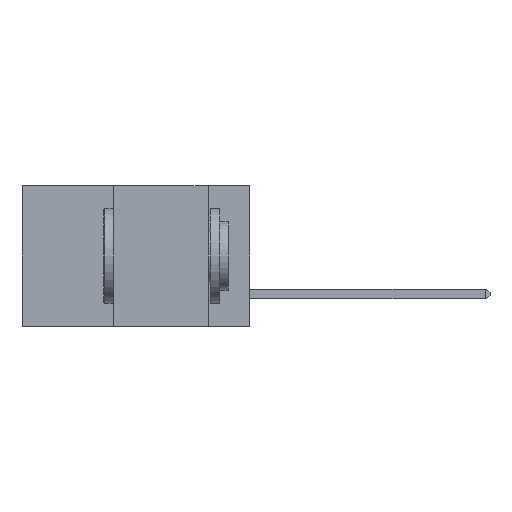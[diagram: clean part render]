
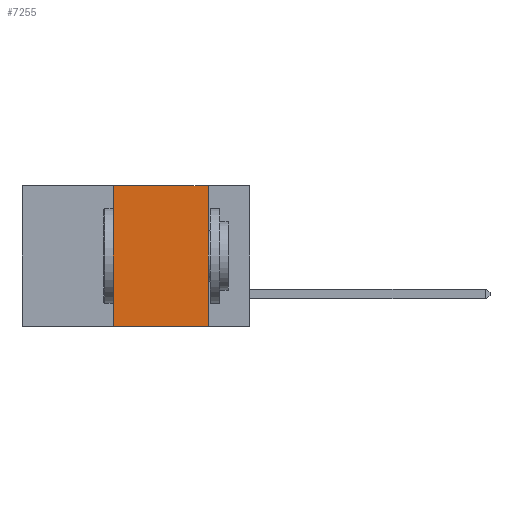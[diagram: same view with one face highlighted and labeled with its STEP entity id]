
A CAD part, left-side view. The second image highlights one B-rep face of the part: STEP entity #7255.
In plain terms, the highlighted planar face has unit normal (-1, 0, 0).
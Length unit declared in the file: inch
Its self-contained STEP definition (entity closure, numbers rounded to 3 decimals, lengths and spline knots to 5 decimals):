
#414 = CARTESIAN_POINT ( 'NONE',  ( 0., 0.11, 0. ) ) ;
#496 = VECTOR ( 'NONE', #1938, 39.37008 ) ;
#1371 = CARTESIAN_POINT ( 'NONE',  ( 0., 0.11, -0.37 ) ) ;
#1938 = DIRECTION ( 'NONE',  ( 0., -1., 0. ) ) ;
#4085 = EDGE_LOOP ( 'NONE', ( #32384, #26216, #20882, #34862 ) ) ;
#5533 = AXIS2_PLACEMENT_3D ( 'NONE', #5590, #24552, #8397 ) ;
#5590 = CARTESIAN_POINT ( 'NONE',  ( 0., 0.6, 0. ) ) ;
#5744 = VECTOR ( 'NONE', #29023, 39.37008 ) ;
#6778 = EDGE_CURVE ( 'NONE', #27101, #29954, #11664, .T. ) ;
#7187 = CARTESIAN_POINT ( 'NONE',  ( 0., 0.36, 0. ) ) ;
#7255 = ADVANCED_FACE ( 'NONE', ( #34595 ), #21906, .F. ) ;
#8397 = DIRECTION ( 'NONE',  ( 0., 0., -1. ) ) ;
#10654 = CARTESIAN_POINT ( 'NONE',  ( 0., 0.36, -0.37 ) ) ;
#11625 = VECTOR ( 'NONE', #34491, 39.37008 ) ;
#11664 = LINE ( 'NONE', #414, #18838 ) ;
#11683 = CARTESIAN_POINT ( 'NONE',  ( 0., 0.11, 0. ) ) ;
#11905 = EDGE_CURVE ( 'NONE', #31286, #27101, #13135, .T. ) ;
#13135 = LINE ( 'NONE', #20959, #5744 ) ;
#15729 = CARTESIAN_POINT ( 'NONE',  ( 0., 0.6, -0.37 ) ) ;
#18838 = VECTOR ( 'NONE', #30053, 39.37008 ) ;
#20882 = ORIENTED_EDGE ( 'NONE', *, *, #34337, .F. ) ;
#20959 = CARTESIAN_POINT ( 'NONE',  ( 0., 0.6, 0. ) ) ;
#21906 = PLANE ( 'NONE',  #5533 ) ;
#24552 = DIRECTION ( 'NONE',  ( 1., 0., 0. ) ) ;
#25136 = VERTEX_POINT ( 'NONE', #10654 ) ;
#26216 = ORIENTED_EDGE ( 'NONE', *, *, #11905, .F. ) ;
#27101 = VERTEX_POINT ( 'NONE', #11683 ) ;
#29023 = DIRECTION ( 'NONE',  ( 0., -1., 0. ) ) ;
#29954 = VERTEX_POINT ( 'NONE', #1371 ) ;
#30053 = DIRECTION ( 'NONE',  ( 0., 0., -1. ) ) ;
#31286 = VERTEX_POINT ( 'NONE', #7187 ) ;
#31848 = CARTESIAN_POINT ( 'NONE',  ( 0., 0.36, 0. ) ) ;
#32384 = ORIENTED_EDGE ( 'NONE', *, *, #6778, .F. ) ;
#32575 = EDGE_CURVE ( 'NONE', #25136, #29954, #34596, .T. ) ;
#32810 = LINE ( 'NONE', #31848, #11625 ) ;
#34337 = EDGE_CURVE ( 'NONE', #25136, #31286, #32810, .T. ) ;
#34491 = DIRECTION ( 'NONE',  ( 0., 0., 1. ) ) ;
#34595 = FACE_OUTER_BOUND ( 'NONE', #4085, .T. ) ;
#34596 = LINE ( 'NONE', #15729, #496 ) ;
#34862 = ORIENTED_EDGE ( 'NONE', *, *, #32575, .T. ) ;
